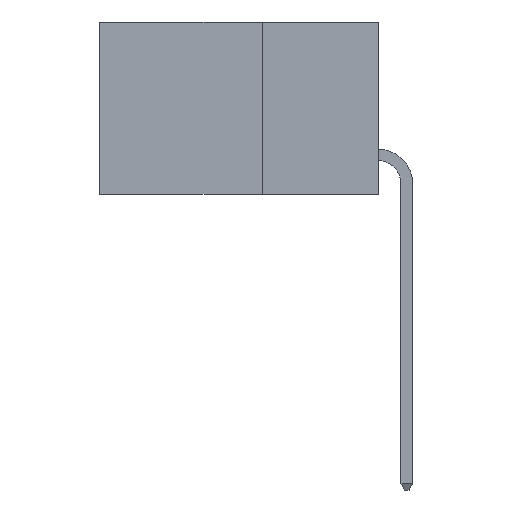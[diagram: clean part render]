
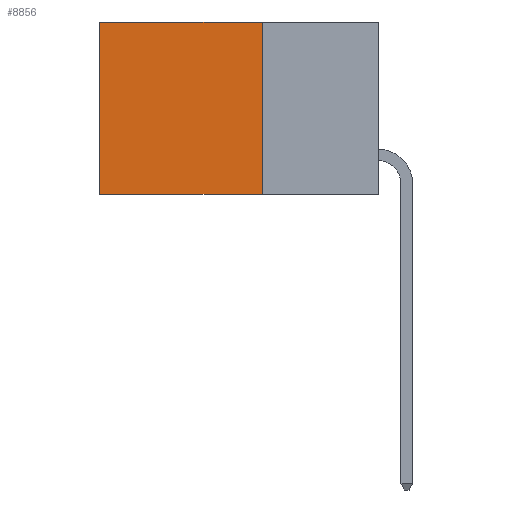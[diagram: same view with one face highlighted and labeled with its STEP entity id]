
A CAD part, left-side view. The second image highlights one B-rep face of the part: STEP entity #8856.
In plain terms, the highlighted planar face has unit normal (-1, 0, 0).
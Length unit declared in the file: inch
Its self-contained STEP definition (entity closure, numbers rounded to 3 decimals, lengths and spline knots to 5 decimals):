
#22 = CARTESIAN_POINT ( 'NONE',  ( 0.2615, 0.25, -0.37 ) ) ;
#642 = EDGE_CURVE ( 'NONE', #4535, #1265, #2019, .T. ) ;
#1265 = VERTEX_POINT ( 'NONE', #5005 ) ;
#2019 = LINE ( 'NONE', #3393, #16426 ) ;
#2829 = LINE ( 'NONE', #22, #17836 ) ;
#3393 = CARTESIAN_POINT ( 'NONE',  ( 0.2615, 0.6, -0.37 ) ) ;
#3716 = EDGE_CURVE ( 'NONE', #21390, #9562, #16911, .T. ) ;
#4535 = VERTEX_POINT ( 'NONE', #11980 ) ;
#4548 = AXIS2_PLACEMENT_3D ( 'NONE', #5776, #9709, #23413 ) ;
#5005 = CARTESIAN_POINT ( 'NONE',  ( 0.2615, 0.6, -0.37 ) ) ;
#5776 = CARTESIAN_POINT ( 'NONE',  ( 0.2615, 0.25, -0.37 ) ) ;
#5973 = VECTOR ( 'NONE', #18590, 39.37008 ) ;
#8856 = ADVANCED_FACE ( 'NONE', ( #11622 ), #21448, .F. ) ;
#9532 = DIRECTION ( 'NONE',  ( 0., 0., -1. ) ) ;
#9562 = VERTEX_POINT ( 'NONE', #24591 ) ;
#9709 = DIRECTION ( 'NONE',  ( 1., 0., 0. ) ) ;
#10942 = ORIENTED_EDGE ( 'NONE', *, *, #18363, .T. ) ;
#11622 = FACE_OUTER_BOUND ( 'NONE', #13945, .T. ) ;
#11980 = CARTESIAN_POINT ( 'NONE',  ( 0.2615, 0.6, 0. ) ) ;
#13945 = EDGE_LOOP ( 'NONE', ( #22142, #14849, #23869, #10942 ) ) ;
#14849 = ORIENTED_EDGE ( 'NONE', *, *, #19338, .F. ) ;
#16426 = VECTOR ( 'NONE', #22262, 39.37008 ) ;
#16605 = CARTESIAN_POINT ( 'NONE',  ( 0.2615, 0.25, 0. ) ) ;
#16911 = LINE ( 'NONE', #21260, #22110 ) ;
#17836 = VECTOR ( 'NONE', #19556, 39.37008 ) ;
#18363 = EDGE_CURVE ( 'NONE', #21390, #4535, #21603, .T. ) ;
#18590 = DIRECTION ( 'NONE',  ( 0., 1., 0. ) ) ;
#19303 = CARTESIAN_POINT ( 'NONE',  ( 0.2615, 0.25, 0. ) ) ;
#19338 = EDGE_CURVE ( 'NONE', #9562, #1265, #2829, .T. ) ;
#19556 = DIRECTION ( 'NONE',  ( 0., 1., 0. ) ) ;
#21260 = CARTESIAN_POINT ( 'NONE',  ( 0.2615, 0.25, -0.37 ) ) ;
#21390 = VERTEX_POINT ( 'NONE', #19303 ) ;
#21448 = PLANE ( 'NONE',  #4548 ) ;
#21603 = LINE ( 'NONE', #16605, #5973 ) ;
#22110 = VECTOR ( 'NONE', #9532, 39.37008 ) ;
#22142 = ORIENTED_EDGE ( 'NONE', *, *, #642, .T. ) ;
#22262 = DIRECTION ( 'NONE',  ( 0., 0., -1. ) ) ;
#23413 = DIRECTION ( 'NONE',  ( 0., 0., -1. ) ) ;
#23869 = ORIENTED_EDGE ( 'NONE', *, *, #3716, .F. ) ;
#24591 = CARTESIAN_POINT ( 'NONE',  ( 0.2615, 0.25, -0.37 ) ) ;
